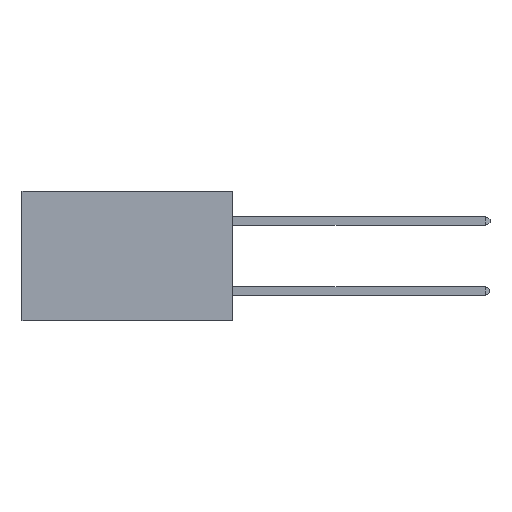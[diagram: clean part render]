
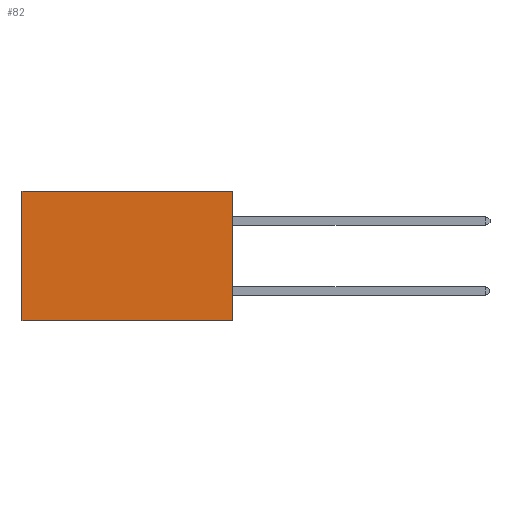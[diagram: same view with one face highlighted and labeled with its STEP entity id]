
A CAD part, left-side view. The second image highlights one B-rep face of the part: STEP entity #82.
In plain terms, the highlighted planar face has unit normal (-1, 0, 0).
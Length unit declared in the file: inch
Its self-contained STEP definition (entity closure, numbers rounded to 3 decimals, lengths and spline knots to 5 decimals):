
#82 = ADVANCED_FACE ( 'NONE', ( #6199 ), #16230, .F. ) ;
#355 = VERTEX_POINT ( 'NONE', #11551 ) ;
#590 = VERTEX_POINT ( 'NONE', #7840 ) ;
#685 = CARTESIAN_POINT ( 'NONE',  ( 0.2875, 0., -0.37 ) ) ;
#827 = ORIENTED_EDGE ( 'NONE', *, *, #5442, .T. ) ;
#1071 = VERTEX_POINT ( 'NONE', #685 ) ;
#1652 = EDGE_LOOP ( 'NONE', ( #827, #2044, #8847, #9642 ) ) ;
#2044 = ORIENTED_EDGE ( 'NONE', *, *, #5247, .F. ) ;
#3030 = EDGE_CURVE ( 'NONE', #590, #355, #4485, .T. ) ;
#3198 = VECTOR ( 'NONE', #13498, 39.37008 ) ;
#4421 = DIRECTION ( 'NONE',  ( 0., 1., 0. ) ) ;
#4485 = LINE ( 'NONE', #12250, #10640 ) ;
#5247 = EDGE_CURVE ( 'NONE', #1071, #11719, #16670, .T. ) ;
#5442 = EDGE_CURVE ( 'NONE', #355, #11719, #13363, .T. ) ;
#6199 = FACE_OUTER_BOUND ( 'NONE', #1652, .T. ) ;
#6414 = VECTOR ( 'NONE', #6942, 39.37008 ) ;
#6484 = CARTESIAN_POINT ( 'NONE',  ( 0.2875, 0., -0.37 ) ) ;
#6666 = LINE ( 'NONE', #9564, #3198 ) ;
#6942 = DIRECTION ( 'NONE',  ( 0., 0., -1. ) ) ;
#7840 = CARTESIAN_POINT ( 'NONE',  ( 0.2875, 0., 0. ) ) ;
#8847 = ORIENTED_EDGE ( 'NONE', *, *, #10562, .F. ) ;
#9291 = VECTOR ( 'NONE', #11720, 39.37008 ) ;
#9564 = CARTESIAN_POINT ( 'NONE',  ( 0.2875, 0., 0. ) ) ;
#9642 = ORIENTED_EDGE ( 'NONE', *, *, #3030, .T. ) ;
#10562 = EDGE_CURVE ( 'NONE', #590, #1071, #6666, .T. ) ;
#10640 = VECTOR ( 'NONE', #4421, 39.37008 ) ;
#11551 = CARTESIAN_POINT ( 'NONE',  ( 0.2875, 0.6, 0. ) ) ;
#11719 = VERTEX_POINT ( 'NONE', #14438 ) ;
#11720 = DIRECTION ( 'NONE',  ( 0., 1., 0. ) ) ;
#12250 = CARTESIAN_POINT ( 'NONE',  ( 0.2875, 0., 0. ) ) ;
#13363 = LINE ( 'NONE', #14762, #6414 ) ;
#13498 = DIRECTION ( 'NONE',  ( 0., 0., -1. ) ) ;
#14438 = CARTESIAN_POINT ( 'NONE',  ( 0.2875, 0.6, -0.37 ) ) ;
#14762 = CARTESIAN_POINT ( 'NONE',  ( 0.2875, 0.6, 0. ) ) ;
#14918 = AXIS2_PLACEMENT_3D ( 'NONE', #16516, #16207, #16170 ) ;
#16170 = DIRECTION ( 'NONE',  ( 0., 0., -1. ) ) ;
#16207 = DIRECTION ( 'NONE',  ( 1., 0., 0. ) ) ;
#16230 = PLANE ( 'NONE',  #14918 ) ;
#16516 = CARTESIAN_POINT ( 'NONE',  ( 0.2875, 0., 0. ) ) ;
#16670 = LINE ( 'NONE', #6484, #9291 ) ;
